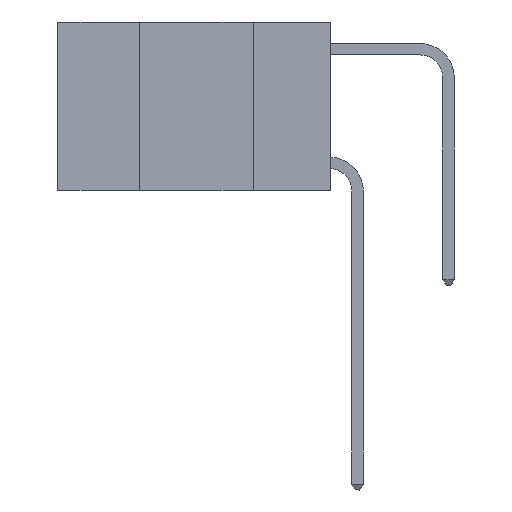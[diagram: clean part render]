
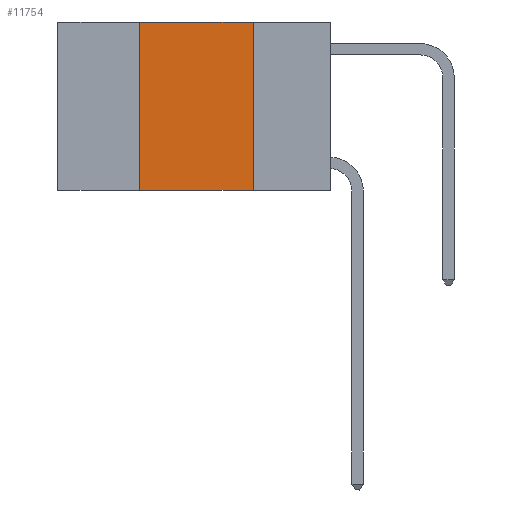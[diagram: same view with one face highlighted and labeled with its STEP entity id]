
A CAD part, left-side view. The second image highlights one B-rep face of the part: STEP entity #11754.
In plain terms, the highlighted planar face has unit normal (-1, 0, 0).
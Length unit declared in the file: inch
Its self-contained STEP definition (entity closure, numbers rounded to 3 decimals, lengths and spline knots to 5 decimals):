
#1045 = ORIENTED_EDGE ( 'NONE', *, *, #25763, .T. ) ;
#1685 = VECTOR ( 'NONE', #3163, 39.37008 ) ;
#1726 = EDGE_LOOP ( 'NONE', ( #25269, #21046, #12273, #1045 ) ) ;
#2101 = CARTESIAN_POINT ( 'NONE',  ( 0., 0.42, 0. ) ) ;
#2181 = VERTEX_POINT ( 'NONE', #26261 ) ;
#3163 = DIRECTION ( 'NONE',  ( 0., 0., -1. ) ) ;
#4915 = LINE ( 'NONE', #19084, #1685 ) ;
#4990 = EDGE_CURVE ( 'NONE', #2181, #15523, #25761, .T. ) ;
#5254 = EDGE_CURVE ( 'NONE', #20843, #15525, #4915, .T. ) ;
#5733 = DIRECTION ( 'NONE',  ( 1., 0., 0. ) ) ;
#8413 = CARTESIAN_POINT ( 'NONE',  ( 0., 0.17, -0.37 ) ) ;
#11754 = ADVANCED_FACE ( 'NONE', ( #15611 ), #12104, .F. ) ;
#11976 = LINE ( 'NONE', #21311, #18784 ) ;
#12104 = PLANE ( 'NONE',  #24254 ) ;
#12273 = ORIENTED_EDGE ( 'NONE', *, *, #4990, .F. ) ;
#12743 = EDGE_CURVE ( 'NONE', #15523, #20843, #11976, .T. ) ;
#13251 = CARTESIAN_POINT ( 'NONE',  ( 0., 0.17, 0. ) ) ;
#13875 = VECTOR ( 'NONE', #24496, 39.37008 ) ;
#15523 = VERTEX_POINT ( 'NONE', #2101 ) ;
#15525 = VERTEX_POINT ( 'NONE', #8413 ) ;
#15611 = FACE_OUTER_BOUND ( 'NONE', #1726, .T. ) ;
#18448 = DIRECTION ( 'NONE',  ( 0., 0., 1. ) ) ;
#18784 = VECTOR ( 'NONE', #23224, 39.37008 ) ;
#19084 = CARTESIAN_POINT ( 'NONE',  ( 0., 0.17, 0. ) ) ;
#20376 = DIRECTION ( 'NONE',  ( 0., 0., -1. ) ) ;
#20843 = VERTEX_POINT ( 'NONE', #13251 ) ;
#21046 = ORIENTED_EDGE ( 'NONE', *, *, #12743, .F. ) ;
#21311 = CARTESIAN_POINT ( 'NONE',  ( 0., 0.6, 0. ) ) ;
#22458 = CARTESIAN_POINT ( 'NONE',  ( 0., 0.6, 0. ) ) ;
#22688 = LINE ( 'NONE', #24320, #13875 ) ;
#23224 = DIRECTION ( 'NONE',  ( 0., -1., 0. ) ) ;
#24254 = AXIS2_PLACEMENT_3D ( 'NONE', #22458, #5733, #20376 ) ;
#24320 = CARTESIAN_POINT ( 'NONE',  ( 0., 0.6, -0.37 ) ) ;
#24496 = DIRECTION ( 'NONE',  ( 0., -1., 0. ) ) ;
#24804 = CARTESIAN_POINT ( 'NONE',  ( 0., 0.42, 0. ) ) ;
#25269 = ORIENTED_EDGE ( 'NONE', *, *, #5254, .F. ) ;
#25761 = LINE ( 'NONE', #24804, #26093 ) ;
#25763 = EDGE_CURVE ( 'NONE', #2181, #15525, #22688, .T. ) ;
#26093 = VECTOR ( 'NONE', #18448, 39.37008 ) ;
#26261 = CARTESIAN_POINT ( 'NONE',  ( 0., 0.42, -0.37 ) ) ;
